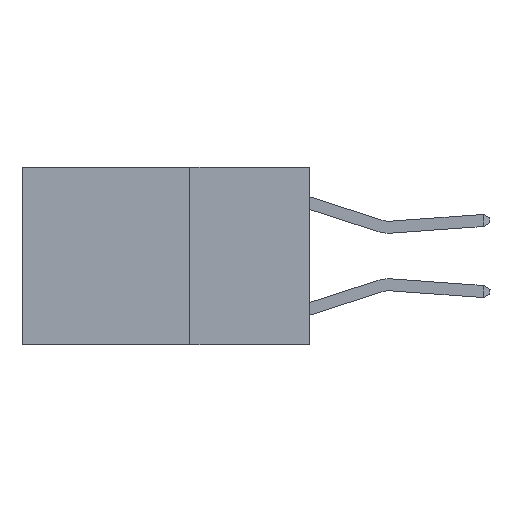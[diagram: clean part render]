
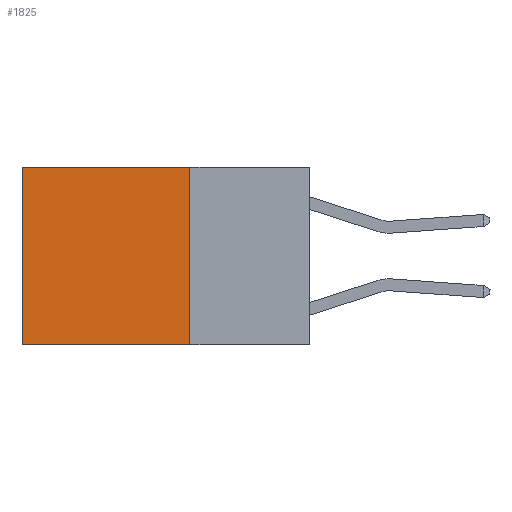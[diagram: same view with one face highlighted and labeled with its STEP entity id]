
A CAD part, left-side view. The second image highlights one B-rep face of the part: STEP entity #1825.
In plain terms, the highlighted planar face has unit normal (-1, 0, 0).
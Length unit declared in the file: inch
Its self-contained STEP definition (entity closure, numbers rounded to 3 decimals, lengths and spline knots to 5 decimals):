
#284 = DIRECTION ( 'NONE',  ( 0., 1., 0. ) ) ;
#310 = EDGE_CURVE ( 'NONE', #6158, #1366, #5514, .T. ) ;
#328 = CARTESIAN_POINT ( 'NONE',  ( 0.2625, 0.25, -0.37 ) ) ;
#384 = DIRECTION ( 'NONE',  ( 1., 0., 0. ) ) ;
#1117 = DIRECTION ( 'NONE',  ( 0., 0., -1. ) ) ;
#1164 = LINE ( 'NONE', #6944, #2708 ) ;
#1167 = FACE_OUTER_BOUND ( 'NONE', #4746, .T. ) ;
#1366 = VERTEX_POINT ( 'NONE', #6907 ) ;
#1463 = VERTEX_POINT ( 'NONE', #5549 ) ;
#1483 = ORIENTED_EDGE ( 'NONE', *, *, #4082, .T. ) ;
#1652 = DIRECTION ( 'NONE',  ( 0., 0., -1. ) ) ;
#1825 = ADVANCED_FACE ( 'NONE', ( #1167 ), #4134, .F. ) ;
#2490 = CARTESIAN_POINT ( 'NONE',  ( 0.2625, 0.25, 0. ) ) ;
#2708 = VECTOR ( 'NONE', #1652, 39.37008 ) ;
#2760 = LINE ( 'NONE', #4885, #5995 ) ;
#2840 = VERTEX_POINT ( 'NONE', #2490 ) ;
#3085 = ORIENTED_EDGE ( 'NONE', *, *, #310, .F. ) ;
#3418 = VECTOR ( 'NONE', #9191, 39.37008 ) ;
#4082 = EDGE_CURVE ( 'NONE', #1463, #1366, #6787, .T. ) ;
#4134 = PLANE ( 'NONE',  #9473 ) ;
#4228 = EDGE_CURVE ( 'NONE', #2840, #6158, #1164, .T. ) ;
#4746 = EDGE_LOOP ( 'NONE', ( #1483, #3085, #5384, #6333 ) ) ;
#4885 = CARTESIAN_POINT ( 'NONE',  ( 0.2625, 0.25, 0. ) ) ;
#5384 = ORIENTED_EDGE ( 'NONE', *, *, #4228, .F. ) ;
#5400 = VECTOR ( 'NONE', #8930, 39.37008 ) ;
#5514 = LINE ( 'NONE', #8900, #5400 ) ;
#5549 = CARTESIAN_POINT ( 'NONE',  ( 0.2625, 0.6, 0. ) ) ;
#5995 = VECTOR ( 'NONE', #284, 39.37008 ) ;
#6158 = VERTEX_POINT ( 'NONE', #328 ) ;
#6333 = ORIENTED_EDGE ( 'NONE', *, *, #7651, .T. ) ;
#6787 = LINE ( 'NONE', #6912, #3418 ) ;
#6907 = CARTESIAN_POINT ( 'NONE',  ( 0.2625, 0.6, -0.37 ) ) ;
#6912 = CARTESIAN_POINT ( 'NONE',  ( 0.2625, 0.6, 0. ) ) ;
#6944 = CARTESIAN_POINT ( 'NONE',  ( 0.2625, 0.25, 0. ) ) ;
#7136 = CARTESIAN_POINT ( 'NONE',  ( 0.2625, 0.25, 0. ) ) ;
#7651 = EDGE_CURVE ( 'NONE', #2840, #1463, #2760, .T. ) ;
#8900 = CARTESIAN_POINT ( 'NONE',  ( 0.2625, 0.25, -0.37 ) ) ;
#8930 = DIRECTION ( 'NONE',  ( 0., 1., 0. ) ) ;
#9191 = DIRECTION ( 'NONE',  ( 0., 0., -1. ) ) ;
#9473 = AXIS2_PLACEMENT_3D ( 'NONE', #7136, #384, #1117 ) ;
